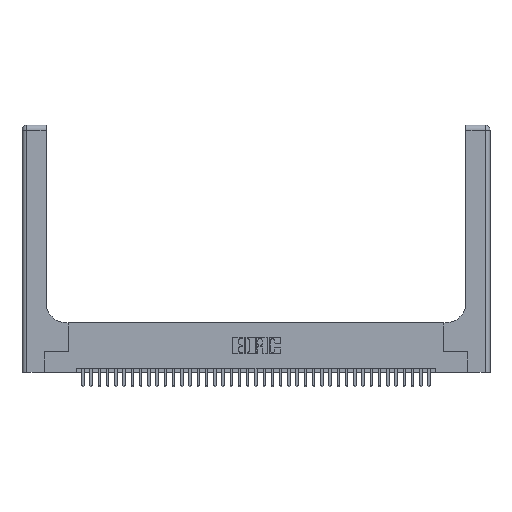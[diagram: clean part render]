
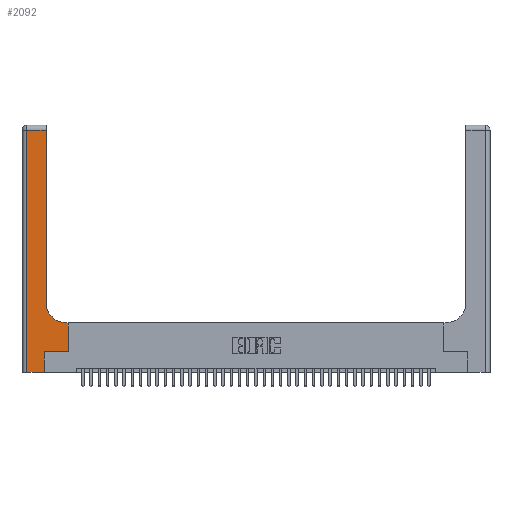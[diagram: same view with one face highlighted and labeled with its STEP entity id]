
A CAD part, top view. The second image highlights one B-rep face of the part: STEP entity #2092.
In plain terms, the highlighted planar face has unit normal (0, 0, 1).
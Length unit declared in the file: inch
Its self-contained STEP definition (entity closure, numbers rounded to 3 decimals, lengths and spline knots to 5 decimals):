
#998 = ORIENTED_EDGE ( 'NONE', *, *, #23312, .T. ) ;
#1581 = LINE ( 'NONE', #13627, #32728 ) ;
#2092 = ADVANCED_FACE ( 'NONE', ( #25269 ), #30027, .F. ) ;
#3416 = VERTEX_POINT ( 'NONE', #23682 ) ;
#3575 = LINE ( 'NONE', #33895, #18692 ) ;
#3834 = LINE ( 'NONE', #10804, #34925 ) ;
#3846 = LINE ( 'NONE', #10324, #9009 ) ;
#4086 = VERTEX_POINT ( 'NONE', #32634 ) ;
#4214 = VECTOR ( 'NONE', #19753, 39.37008 ) ;
#4777 = ORIENTED_EDGE ( 'NONE', *, *, #8876, .T. ) ;
#5091 = CARTESIAN_POINT ( 'NONE',  ( 0.5415, 0.6, 0.37 ) ) ;
#5409 = DIRECTION ( 'NONE',  ( -1., 0., 0. ) ) ;
#5690 = ORIENTED_EDGE ( 'NONE', *, *, #27565, .T. ) ;
#6669 = EDGE_CURVE ( 'NONE', #22094, #12196, #3575, .T. ) ;
#7395 = LINE ( 'NONE', #20924, #30563 ) ;
#7522 = CARTESIAN_POINT ( 'NONE',  ( 0.5585, 0.25, 0.37 ) ) ;
#8843 = VERTEX_POINT ( 'NONE', #7522 ) ;
#8876 = EDGE_CURVE ( 'NONE', #8843, #4086, #1581, .T. ) ;
#9001 = EDGE_CURVE ( 'NONE', #18272, #22940, #13836, .T. ) ;
#9009 = VECTOR ( 'NONE', #31442, 39.37008 ) ;
#9688 = ORIENTED_EDGE ( 'NONE', *, *, #36534, .T. ) ;
#10186 = ORIENTED_EDGE ( 'NONE', *, *, #35502, .T. ) ;
#10324 = CARTESIAN_POINT ( 'NONE',  ( 0.2915, 0.6, 0.37 ) ) ;
#10615 = CARTESIAN_POINT ( 'NONE',  ( 0.2915, 3., 0.37 ) ) ;
#10804 = CARTESIAN_POINT ( 'NONE',  ( 0.269, 0., 0.37 ) ) ;
#11273 = EDGE_CURVE ( 'NONE', #16014, #31460, #27284, .T. ) ;
#11955 = CARTESIAN_POINT ( 'NONE',  ( 0., 3., 0.37 ) ) ;
#11976 = CARTESIAN_POINT ( 'NONE',  ( 0.06, 0., 0.37 ) ) ;
#12196 = VERTEX_POINT ( 'NONE', #30648 ) ;
#12689 = AXIS2_PLACEMENT_3D ( 'NONE', #13158, #34223, #16197 ) ;
#12730 = VECTOR ( 'NONE', #18108, 39.37008 ) ;
#13158 = CARTESIAN_POINT ( 'NONE',  ( 0.5415, 0.85, 0.37 ) ) ;
#13627 = CARTESIAN_POINT ( 'NONE',  ( 0.5585, 0.25, 0.37 ) ) ;
#13836 = LINE ( 'NONE', #29186, #28951 ) ;
#14004 = AXIS2_PLACEMENT_3D ( 'NONE', #11955, #36003, #18004 ) ;
#14632 = EDGE_CURVE ( 'NONE', #4086, #16014, #3846, .T. ) ;
#15075 = CARTESIAN_POINT ( 'NONE',  ( 0.06, 3., 0.37 ) ) ;
#15703 = ORIENTED_EDGE ( 'NONE', *, *, #9001, .T. ) ;
#16014 = VERTEX_POINT ( 'NONE', #5091 ) ;
#16197 = DIRECTION ( 'NONE',  ( 1., 0., 0. ) ) ;
#16943 = LINE ( 'NONE', #15075, #12730 ) ;
#18004 = DIRECTION ( 'NONE',  ( -1., 0., 0. ) ) ;
#18108 = DIRECTION ( 'NONE',  ( 0., -1., 0. ) ) ;
#18272 = VERTEX_POINT ( 'NONE', #20835 ) ;
#18692 = VECTOR ( 'NONE', #18889, 39.37008 ) ;
#18889 = DIRECTION ( 'NONE',  ( 1., 0., 0. ) ) ;
#19753 = DIRECTION ( 'NONE',  ( 0., 1., 0. ) ) ;
#20600 = EDGE_LOOP ( 'NONE', ( #9688, #15703, #10186, #31433, #5690, #998, #4777, #36090, #29975 ) ) ;
#20835 = CARTESIAN_POINT ( 'NONE',  ( 0.2915, 2.94, 0.37 ) ) ;
#20924 = CARTESIAN_POINT ( 'NONE',  ( 0.269, 0.25, 0.37 ) ) ;
#22094 = VERTEX_POINT ( 'NONE', #11976 ) ;
#22940 = VERTEX_POINT ( 'NONE', #31176 ) ;
#23312 = EDGE_CURVE ( 'NONE', #3416, #8843, #7395, .T. ) ;
#23682 = CARTESIAN_POINT ( 'NONE',  ( 0.269, 0.25, 0.37 ) ) ;
#23996 = DIRECTION ( 'NONE',  ( 1., 0., 0. ) ) ;
#25269 = FACE_OUTER_BOUND ( 'NONE', #20600, .T. ) ;
#27284 = CIRCLE ( 'NONE', #12689, 0.25 ) ;
#27406 = LINE ( 'NONE', #10615, #4214 ) ;
#27565 = EDGE_CURVE ( 'NONE', #12196, #3416, #3834, .T. ) ;
#28951 = VECTOR ( 'NONE', #5409, 39.37008 ) ;
#29186 = CARTESIAN_POINT ( 'NONE',  ( 0., 2.94, 0.37 ) ) ;
#29975 = ORIENTED_EDGE ( 'NONE', *, *, #11273, .T. ) ;
#30027 = PLANE ( 'NONE',  #14004 ) ;
#30563 = VECTOR ( 'NONE', #23996, 39.37008 ) ;
#30648 = CARTESIAN_POINT ( 'NONE',  ( 0.269, 0., 0.37 ) ) ;
#31176 = CARTESIAN_POINT ( 'NONE',  ( 0.06, 2.94, 0.37 ) ) ;
#31433 = ORIENTED_EDGE ( 'NONE', *, *, #6669, .T. ) ;
#31442 = DIRECTION ( 'NONE',  ( -1., 0., 0. ) ) ;
#31460 = VERTEX_POINT ( 'NONE', #37918 ) ;
#32634 = CARTESIAN_POINT ( 'NONE',  ( 0.5585, 0.6, 0.37 ) ) ;
#32728 = VECTOR ( 'NONE', #37622, 39.37008 ) ;
#33895 = CARTESIAN_POINT ( 'NONE',  ( 0., 0., 0.37 ) ) ;
#34223 = DIRECTION ( 'NONE',  ( 0., 0., -1. ) ) ;
#34925 = VECTOR ( 'NONE', #37861, 39.37008 ) ;
#35502 = EDGE_CURVE ( 'NONE', #22940, #22094, #16943, .T. ) ;
#36003 = DIRECTION ( 'NONE',  ( 0., 0., -1. ) ) ;
#36090 = ORIENTED_EDGE ( 'NONE', *, *, #14632, .T. ) ;
#36534 = EDGE_CURVE ( 'NONE', #31460, #18272, #27406, .T. ) ;
#37622 = DIRECTION ( 'NONE',  ( 0., 1., 0. ) ) ;
#37861 = DIRECTION ( 'NONE',  ( 0., 1., 0. ) ) ;
#37918 = CARTESIAN_POINT ( 'NONE',  ( 0.2915, 0.85, 0.37 ) ) ;
